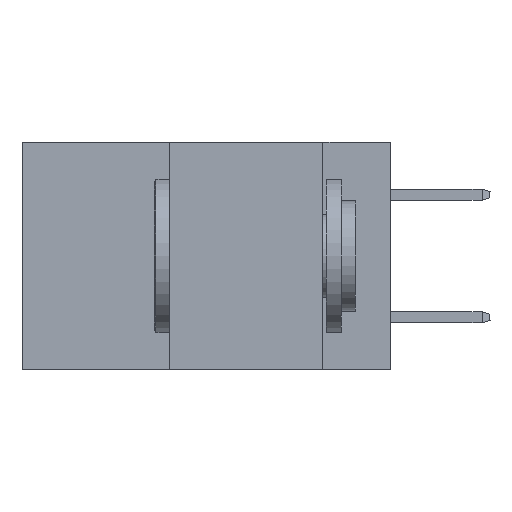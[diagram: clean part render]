
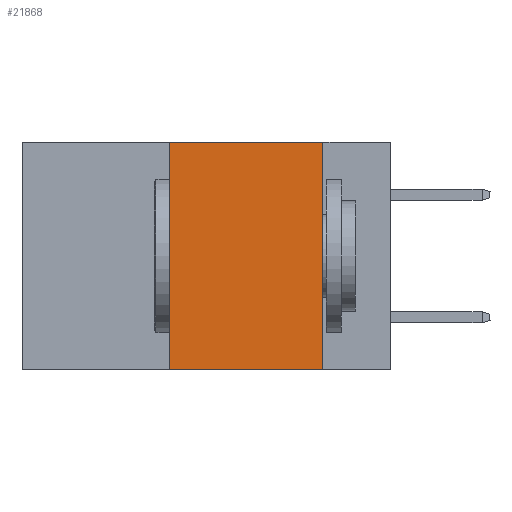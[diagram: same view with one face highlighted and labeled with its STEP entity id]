
A CAD part, left-side view. The second image highlights one B-rep face of the part: STEP entity #21868.
In plain terms, the highlighted planar face has unit normal (-1, 0, 0).
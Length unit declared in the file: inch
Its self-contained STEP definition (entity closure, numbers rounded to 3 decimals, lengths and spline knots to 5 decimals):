
#664 = VERTEX_POINT ( 'NONE', #30451 ) ;
#954 = VECTOR ( 'NONE', #17456, 39.37008 ) ;
#1860 = LINE ( 'NONE', #12006, #954 ) ;
#2037 = EDGE_CURVE ( 'NONE', #26122, #8080, #1860, .T. ) ;
#2920 = FACE_OUTER_BOUND ( 'NONE', #10728, .T. ) ;
#3744 = LINE ( 'NONE', #23603, #32202 ) ;
#5077 = CARTESIAN_POINT ( 'NONE',  ( 0., 0.36, 0. ) ) ;
#6885 = DIRECTION ( 'NONE',  ( 1., 0., 0. ) ) ;
#6942 = EDGE_CURVE ( 'NONE', #13848, #26122, #19876, .T. ) ;
#8080 = VERTEX_POINT ( 'NONE', #24977 ) ;
#10728 = EDGE_LOOP ( 'NONE', ( #13041, #28609, #23457, #31582 ) ) ;
#12006 = CARTESIAN_POINT ( 'NONE',  ( 0., 0.6, 0. ) ) ;
#13041 = ORIENTED_EDGE ( 'NONE', *, *, #13187, .F. ) ;
#13187 = EDGE_CURVE ( 'NONE', #8080, #664, #28410, .T. ) ;
#13848 = VERTEX_POINT ( 'NONE', #19154 ) ;
#15253 = CARTESIAN_POINT ( 'NONE',  ( 0., 0.36, 0. ) ) ;
#17456 = DIRECTION ( 'NONE',  ( 0., -1., 0. ) ) ;
#18161 = DIRECTION ( 'NONE',  ( 0., -1., 0. ) ) ;
#18835 = CARTESIAN_POINT ( 'NONE',  ( 0., 0.11, 0. ) ) ;
#18959 = DIRECTION ( 'NONE',  ( 0., 0., -1. ) ) ;
#19154 = CARTESIAN_POINT ( 'NONE',  ( 0., 0.36, -0.37 ) ) ;
#19876 = LINE ( 'NONE', #15253, #26371 ) ;
#21090 = VECTOR ( 'NONE', #18959, 39.37008 ) ;
#21868 = ADVANCED_FACE ( 'NONE', ( #2920 ), #23330, .F. ) ;
#23330 = PLANE ( 'NONE',  #26188 ) ;
#23457 = ORIENTED_EDGE ( 'NONE', *, *, #6942, .F. ) ;
#23603 = CARTESIAN_POINT ( 'NONE',  ( 0., 0.6, -0.37 ) ) ;
#24977 = CARTESIAN_POINT ( 'NONE',  ( 0., 0.11, 0. ) ) ;
#26122 = VERTEX_POINT ( 'NONE', #5077 ) ;
#26188 = AXIS2_PLACEMENT_3D ( 'NONE', #34261, #6885, #26256 ) ;
#26256 = DIRECTION ( 'NONE',  ( 0., 0., -1. ) ) ;
#26371 = VECTOR ( 'NONE', #29016, 39.37008 ) ;
#28410 = LINE ( 'NONE', #18835, #21090 ) ;
#28609 = ORIENTED_EDGE ( 'NONE', *, *, #2037, .F. ) ;
#29016 = DIRECTION ( 'NONE',  ( 0., 0., 1. ) ) ;
#30451 = CARTESIAN_POINT ( 'NONE',  ( 0., 0.11, -0.37 ) ) ;
#31582 = ORIENTED_EDGE ( 'NONE', *, *, #32743, .T. ) ;
#32202 = VECTOR ( 'NONE', #18161, 39.37008 ) ;
#32743 = EDGE_CURVE ( 'NONE', #13848, #664, #3744, .T. ) ;
#34261 = CARTESIAN_POINT ( 'NONE',  ( 0., 0.6, 0. ) ) ;
